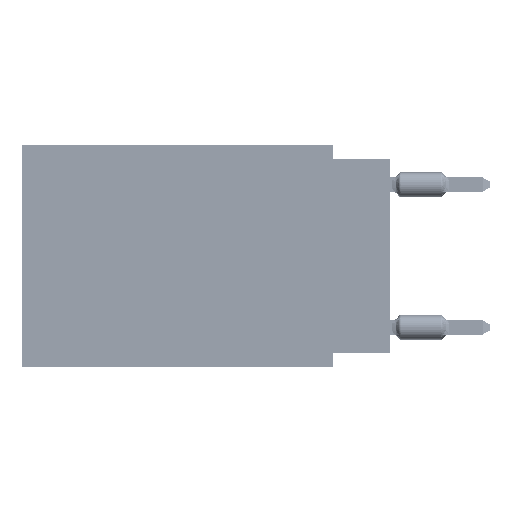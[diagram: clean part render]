
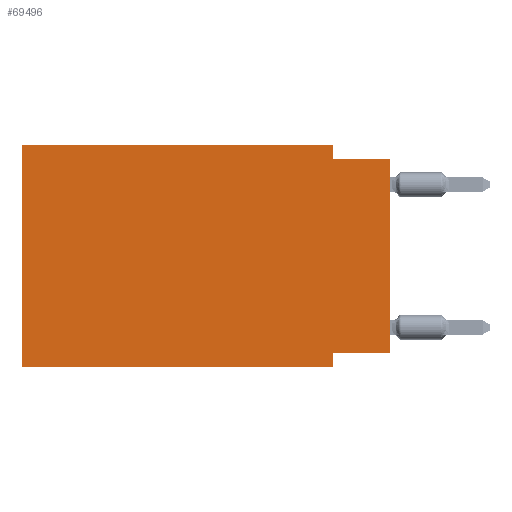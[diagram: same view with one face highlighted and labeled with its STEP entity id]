
A CAD part, left-side view. The second image highlights one B-rep face of the part: STEP entity #69496.
In plain terms, the highlighted planar face has unit normal (-1, 0, 0).
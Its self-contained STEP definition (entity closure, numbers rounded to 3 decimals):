
#387 = VERTEX_POINT ( 'NONE', #16871 ) ;
#511 = LINE ( 'NONE', #60868, #59085 ) ;
#5313 = PLANE ( 'NONE',  #6450 ) ;
#6352 = VERTEX_POINT ( 'NONE', #12834 ) ;
#6450 = AXIS2_PLACEMENT_3D ( 'NONE', #54478, #29701, #30894 ) ;
#6625 = EDGE_CURVE ( 'NONE', #53652, #45266, #22754, .T. ) ;
#10707 = EDGE_CURVE ( 'NONE', #27273, #6352, #17940, .T. ) ;
#10760 = CARTESIAN_POINT ( 'NONE',  ( 0., 16.383, -9.906 ) ) ;
#12834 = CARTESIAN_POINT ( 'NONE',  ( 0., 0., -0.635 ) ) ;
#13914 = DIRECTION ( 'NONE',  ( 0., 0., 1. ) ) ;
#14532 = VERTEX_POINT ( 'NONE', #26948 ) ;
#14610 = ORIENTED_EDGE ( 'NONE', *, *, #26039, .F. ) ;
#14686 = EDGE_CURVE ( 'NONE', #16702, #45266, #78089, .T. ) ;
#14772 = DIRECTION ( 'NONE',  ( 0., -1., 0. ) ) ;
#14991 = VECTOR ( 'NONE', #13914, 1000. ) ;
#15921 = EDGE_LOOP ( 'NONE', ( #25934, #42523, #14610, #45083, #78355, #16686, #71740, #46799 ) ) ;
#16686 = ORIENTED_EDGE ( 'NONE', *, *, #6625, .T. ) ;
#16702 = VERTEX_POINT ( 'NONE', #38792 ) ;
#16871 = CARTESIAN_POINT ( 'NONE',  ( 0., 2.54, 0. ) ) ;
#17321 = VECTOR ( 'NONE', #37137, 1000. ) ;
#17940 = LINE ( 'NONE', #47932, #17321 ) ;
#18689 = DIRECTION ( 'NONE',  ( 0., -1., 0. ) ) ;
#19358 = LINE ( 'NONE', #25752, #53774 ) ;
#19514 = CARTESIAN_POINT ( 'NONE',  ( 0., 16.383, 0. ) ) ;
#19864 = LINE ( 'NONE', #73476, #34206 ) ;
#22754 = LINE ( 'NONE', #10760, #57696 ) ;
#24531 = VERTEX_POINT ( 'NONE', #33973 ) ;
#25752 = CARTESIAN_POINT ( 'NONE',  ( 0., 0., -9.271 ) ) ;
#25934 = ORIENTED_EDGE ( 'NONE', *, *, #10707, .T. ) ;
#26039 = EDGE_CURVE ( 'NONE', #387, #24531, #511, .T. ) ;
#26948 = CARTESIAN_POINT ( 'NONE',  ( 0., 16.383, 0. ) ) ;
#27273 = VERTEX_POINT ( 'NONE', #50463 ) ;
#28144 = DIRECTION ( 'NONE',  ( 0., 0., -1. ) ) ;
#29701 = DIRECTION ( 'NONE',  ( 1., 0., 0. ) ) ;
#30894 = DIRECTION ( 'NONE',  ( 0., 0., -1. ) ) ;
#32128 = CARTESIAN_POINT ( 'NONE',  ( 0., 16.383, -9.906 ) ) ;
#33973 = CARTESIAN_POINT ( 'NONE',  ( 0., 2.54, -0.635 ) ) ;
#34206 = VECTOR ( 'NONE', #18689, 1000. ) ;
#35157 = DIRECTION ( 'NONE',  ( 0., -1., 0. ) ) ;
#35315 = CARTESIAN_POINT ( 'NONE',  ( 0., 2.54, -9.906 ) ) ;
#37137 = DIRECTION ( 'NONE',  ( 0., 0., 1. ) ) ;
#38792 = CARTESIAN_POINT ( 'NONE',  ( 0., 2.54, -9.271 ) ) ;
#40168 = VECTOR ( 'NONE', #14772, 1000. ) ;
#42523 = ORIENTED_EDGE ( 'NONE', *, *, #62247, .F. ) ;
#42587 = EDGE_CURVE ( 'NONE', #27273, #16702, #19358, .T. ) ;
#43280 = DIRECTION ( 'NONE',  ( 0., 0., -1. ) ) ;
#43763 = DIRECTION ( 'NONE',  ( 0., 1., 0. ) ) ;
#45083 = ORIENTED_EDGE ( 'NONE', *, *, #65962, .F. ) ;
#45266 = VERTEX_POINT ( 'NONE', #53868 ) ;
#46799 = ORIENTED_EDGE ( 'NONE', *, *, #42587, .F. ) ;
#47932 = CARTESIAN_POINT ( 'NONE',  ( 0., 0., 0. ) ) ;
#50101 = EDGE_CURVE ( 'NONE', #53652, #14532, #74300, .T. ) ;
#50463 = CARTESIAN_POINT ( 'NONE',  ( 0., 0., -9.271 ) ) ;
#53652 = VERTEX_POINT ( 'NONE', #32128 ) ;
#53774 = VECTOR ( 'NONE', #43763, 1000. ) ;
#53868 = CARTESIAN_POINT ( 'NONE',  ( 0., 2.54, -9.906 ) ) ;
#54478 = CARTESIAN_POINT ( 'NONE',  ( 0., 16.383, 0. ) ) ;
#55559 = VECTOR ( 'NONE', #28144, 1000. ) ;
#57696 = VECTOR ( 'NONE', #35157, 1000. ) ;
#59085 = VECTOR ( 'NONE', #43280, 1000. ) ;
#60868 = CARTESIAN_POINT ( 'NONE',  ( 0., 2.54, 0. ) ) ;
#62247 = EDGE_CURVE ( 'NONE', #24531, #6352, #69553, .T. ) ;
#65962 = EDGE_CURVE ( 'NONE', #14532, #387, #19864, .T. ) ;
#68761 = CARTESIAN_POINT ( 'NONE',  ( 0., 0., -0.635 ) ) ;
#69496 = ADVANCED_FACE ( 'NONE', ( #74074 ), #5313, .F. ) ;
#69553 = LINE ( 'NONE', #68761, #40168 ) ;
#71740 = ORIENTED_EDGE ( 'NONE', *, *, #14686, .F. ) ;
#73476 = CARTESIAN_POINT ( 'NONE',  ( 0., 16.383, 0. ) ) ;
#74074 = FACE_OUTER_BOUND ( 'NONE', #15921, .T. ) ;
#74300 = LINE ( 'NONE', #19514, #14991 ) ;
#78089 = LINE ( 'NONE', #35315, #55559 ) ;
#78355 = ORIENTED_EDGE ( 'NONE', *, *, #50101, .F. ) ;
